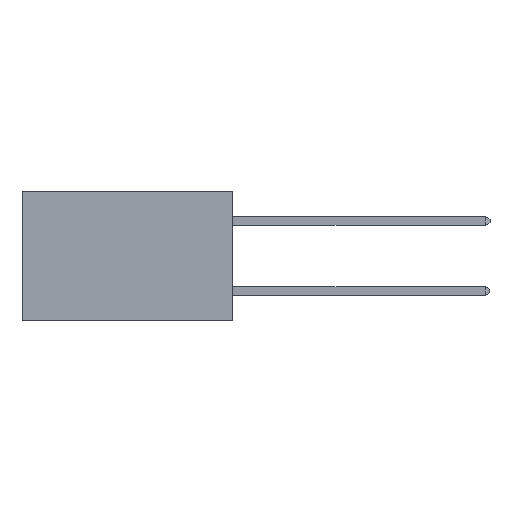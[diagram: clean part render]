
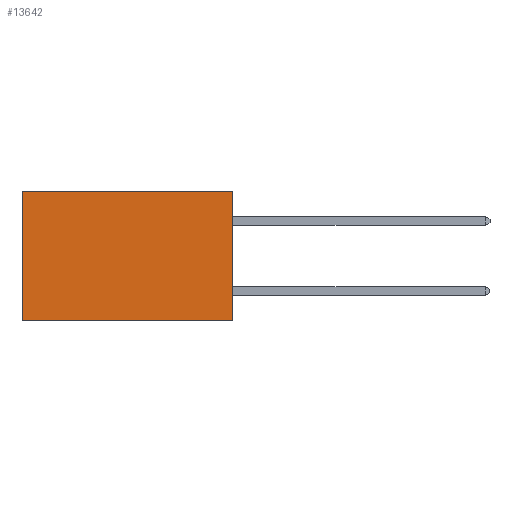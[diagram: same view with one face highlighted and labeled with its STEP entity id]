
A CAD part, left-side view. The second image highlights one B-rep face of the part: STEP entity #13642.
In plain terms, the highlighted planar face has unit normal (-1, 0, 0).
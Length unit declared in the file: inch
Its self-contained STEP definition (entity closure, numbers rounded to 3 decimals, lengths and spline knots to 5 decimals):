
#739 = DIRECTION ( 'NONE',  ( 0., 0., -1. ) ) ;
#1128 = CARTESIAN_POINT ( 'NONE',  ( 0.2875, 0., -0.37 ) ) ;
#1402 = CARTESIAN_POINT ( 'NONE',  ( 0.2875, 0., -0.37 ) ) ;
#1452 = LINE ( 'NONE', #13048, #10757 ) ;
#2772 = VECTOR ( 'NONE', #3634, 39.37008 ) ;
#3400 = LINE ( 'NONE', #5995, #9845 ) ;
#3634 = DIRECTION ( 'NONE',  ( 0., 0., -1. ) ) ;
#3768 = VERTEX_POINT ( 'NONE', #9123 ) ;
#4109 = CARTESIAN_POINT ( 'NONE',  ( 0.2875, 0.6, 0. ) ) ;
#4345 = ORIENTED_EDGE ( 'NONE', *, *, #6291, .F. ) ;
#4812 = CARTESIAN_POINT ( 'NONE',  ( 0.2875, 0.6, 0. ) ) ;
#5018 = AXIS2_PLACEMENT_3D ( 'NONE', #11642, #8019, #739 ) ;
#5995 = CARTESIAN_POINT ( 'NONE',  ( 0.2875, 0., 0. ) ) ;
#6041 = CARTESIAN_POINT ( 'NONE',  ( 0.2875, 0., 0. ) ) ;
#6126 = ORIENTED_EDGE ( 'NONE', *, *, #6837, .F. ) ;
#6291 = EDGE_CURVE ( 'NONE', #11922, #3768, #11421, .T. ) ;
#6769 = PLANE ( 'NONE',  #5018 ) ;
#6837 = EDGE_CURVE ( 'NONE', #9900, #11922, #3400, .T. ) ;
#6964 = DIRECTION ( 'NONE',  ( 0., 1., 0. ) ) ;
#7219 = DIRECTION ( 'NONE',  ( 0., 0., -1. ) ) ;
#8019 = DIRECTION ( 'NONE',  ( 1., 0., 0. ) ) ;
#8535 = EDGE_CURVE ( 'NONE', #8795, #3768, #9990, .T. ) ;
#8795 = VERTEX_POINT ( 'NONE', #4109 ) ;
#9123 = CARTESIAN_POINT ( 'NONE',  ( 0.2875, 0.6, -0.37 ) ) ;
#9845 = VECTOR ( 'NONE', #7219, 39.37008 ) ;
#9900 = VERTEX_POINT ( 'NONE', #6041 ) ;
#9951 = FACE_OUTER_BOUND ( 'NONE', #13997, .T. ) ;
#9990 = LINE ( 'NONE', #4812, #2772 ) ;
#10757 = VECTOR ( 'NONE', #6964, 39.37008 ) ;
#11421 = LINE ( 'NONE', #1402, #14135 ) ;
#11642 = CARTESIAN_POINT ( 'NONE',  ( 0.2875, 0., 0. ) ) ;
#11922 = VERTEX_POINT ( 'NONE', #1128 ) ;
#12333 = DIRECTION ( 'NONE',  ( 0., 1., 0. ) ) ;
#12407 = EDGE_CURVE ( 'NONE', #9900, #8795, #1452, .T. ) ;
#12904 = ORIENTED_EDGE ( 'NONE', *, *, #8535, .T. ) ;
#13048 = CARTESIAN_POINT ( 'NONE',  ( 0.2875, 0., 0. ) ) ;
#13642 = ADVANCED_FACE ( 'NONE', ( #9951 ), #6769, .F. ) ;
#13997 = EDGE_LOOP ( 'NONE', ( #12904, #4345, #6126, #15458 ) ) ;
#14135 = VECTOR ( 'NONE', #12333, 39.37008 ) ;
#15458 = ORIENTED_EDGE ( 'NONE', *, *, #12407, .T. ) ;
